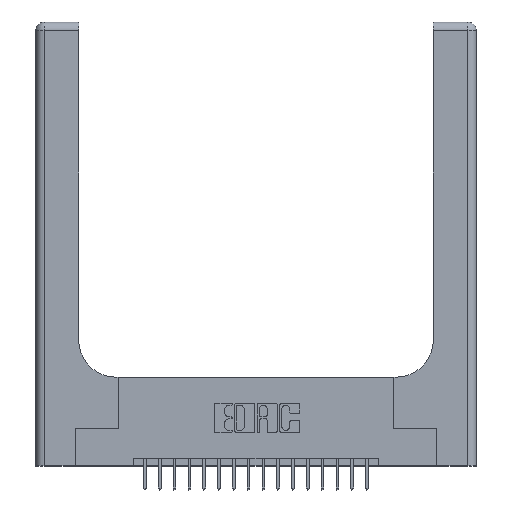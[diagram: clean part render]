
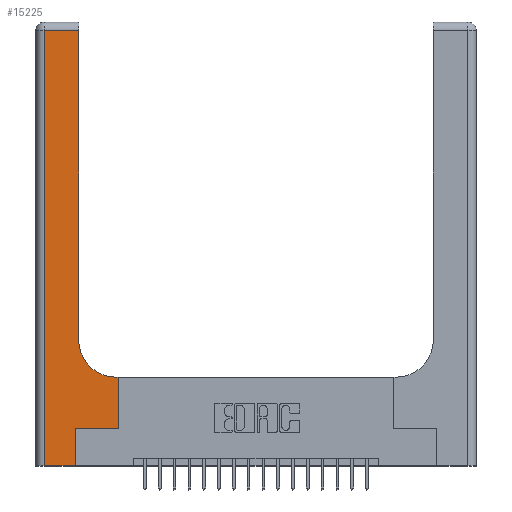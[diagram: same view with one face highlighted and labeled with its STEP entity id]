
A CAD part, top view. The second image highlights one B-rep face of the part: STEP entity #15225.
In plain terms, the highlighted planar face has unit normal (0, 0, 1).
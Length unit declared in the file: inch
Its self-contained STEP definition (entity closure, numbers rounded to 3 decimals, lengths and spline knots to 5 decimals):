
#48 = LINE ( 'NONE', #157, #8401 ) ;
#157 = CARTESIAN_POINT ( 'NONE',  ( 0.06, 3., 0.37 ) ) ;
#583 = CARTESIAN_POINT ( 'NONE',  ( 0.5415, 0.85, 0.37 ) ) ;
#613 = VERTEX_POINT ( 'NONE', #3987 ) ;
#1286 = LINE ( 'NONE', #4008, #18329 ) ;
#1529 = DIRECTION ( 'NONE',  ( 0., 1., 0. ) ) ;
#1548 = CARTESIAN_POINT ( 'NONE',  ( 0.5585, 0.25, 0.37 ) ) ;
#1689 = EDGE_CURVE ( 'NONE', #8178, #613, #48, .T. ) ;
#1707 = AXIS2_PLACEMENT_3D ( 'NONE', #583, #12225, #2245 ) ;
#1746 = CARTESIAN_POINT ( 'NONE',  ( 0., 0., 0.37 ) ) ;
#1817 = DIRECTION ( 'NONE',  ( 0., -1., 0. ) ) ;
#2245 = DIRECTION ( 'NONE',  ( 1., 0., 0. ) ) ;
#2800 = LINE ( 'NONE', #5337, #7235 ) ;
#2855 = EDGE_CURVE ( 'NONE', #16870, #15335, #6807, .T. ) ;
#3178 = CARTESIAN_POINT ( 'NONE',  ( 0.269, 0., 0.37 ) ) ;
#3323 = VECTOR ( 'NONE', #11579, 39.37008 ) ;
#3483 = DIRECTION ( 'NONE',  ( 1., 0., 0. ) ) ;
#3987 = CARTESIAN_POINT ( 'NONE',  ( 0.06, 0., 0.37 ) ) ;
#4008 = CARTESIAN_POINT ( 'NONE',  ( 0.269, 0.25, 0.37 ) ) ;
#4037 = CARTESIAN_POINT ( 'NONE',  ( 0., 3., 0.37 ) ) ;
#4660 = ORIENTED_EDGE ( 'NONE', *, *, #11950, .T. ) ;
#4799 = EDGE_CURVE ( 'NONE', #21310, #8178, #2800, .T. ) ;
#4954 = VERTEX_POINT ( 'NONE', #13936 ) ;
#5124 = ORIENTED_EDGE ( 'NONE', *, *, #17479, .T. ) ;
#5203 = EDGE_CURVE ( 'NONE', #12204, #17050, #15938, .T. ) ;
#5283 = ORIENTED_EDGE ( 'NONE', *, *, #5203, .T. ) ;
#5337 = CARTESIAN_POINT ( 'NONE',  ( 0., 2.94, 0.37 ) ) ;
#5670 = DIRECTION ( 'NONE',  ( 1., 0., 0. ) ) ;
#5701 = PLANE ( 'NONE',  #16734 ) ;
#5713 = CARTESIAN_POINT ( 'NONE',  ( 0.5585, 0.25, 0.37 ) ) ;
#6283 = VECTOR ( 'NONE', #11266, 39.37008 ) ;
#6622 = CARTESIAN_POINT ( 'NONE',  ( 0.2915, 2.94, 0.37 ) ) ;
#6807 = LINE ( 'NONE', #20992, #6283 ) ;
#7235 = VECTOR ( 'NONE', #18490, 39.37008 ) ;
#7390 = DIRECTION ( 'NONE',  ( 0., 0., -1. ) ) ;
#7600 = ORIENTED_EDGE ( 'NONE', *, *, #18216, .T. ) ;
#8178 = VERTEX_POINT ( 'NONE', #20982 ) ;
#8401 = VECTOR ( 'NONE', #1817, 39.37008 ) ;
#8454 = FACE_OUTER_BOUND ( 'NONE', #10889, .T. ) ;
#8678 = VERTEX_POINT ( 'NONE', #5713 ) ;
#9016 = VECTOR ( 'NONE', #14799, 39.37008 ) ;
#9819 = ORIENTED_EDGE ( 'NONE', *, *, #4799, .T. ) ;
#10201 = CARTESIAN_POINT ( 'NONE',  ( 0.5415, 0.6, 0.37 ) ) ;
#10423 = VECTOR ( 'NONE', #1529, 39.37008 ) ;
#10822 = VECTOR ( 'NONE', #3483, 39.37008 ) ;
#10889 = EDGE_LOOP ( 'NONE', ( #5124, #9819, #11384, #4660, #15457, #7600, #12024, #5283, #13872 ) ) ;
#11266 = DIRECTION ( 'NONE',  ( 0., 1., 0. ) ) ;
#11384 = ORIENTED_EDGE ( 'NONE', *, *, #1689, .T. ) ;
#11513 = CARTESIAN_POINT ( 'NONE',  ( 0.2915, 3., 0.37 ) ) ;
#11579 = DIRECTION ( 'NONE',  ( -1., 0., 0. ) ) ;
#11859 = EDGE_CURVE ( 'NONE', #8678, #12204, #21021, .T. ) ;
#11950 = EDGE_CURVE ( 'NONE', #613, #16870, #19522, .T. ) ;
#12024 = ORIENTED_EDGE ( 'NONE', *, *, #11859, .T. ) ;
#12204 = VERTEX_POINT ( 'NONE', #20376 ) ;
#12225 = DIRECTION ( 'NONE',  ( 0., 0., -1. ) ) ;
#12425 = CIRCLE ( 'NONE', #1707, 0.25 ) ;
#12588 = CARTESIAN_POINT ( 'NONE',  ( 0.269, 0.25, 0.37 ) ) ;
#13872 = ORIENTED_EDGE ( 'NONE', *, *, #19265, .T. ) ;
#13936 = CARTESIAN_POINT ( 'NONE',  ( 0.2915, 0.85, 0.37 ) ) ;
#14282 = LINE ( 'NONE', #11513, #10423 ) ;
#14799 = DIRECTION ( 'NONE',  ( 0., 1., 0. ) ) ;
#15225 = ADVANCED_FACE ( 'NONE', ( #8454 ), #5701, .F. ) ;
#15335 = VERTEX_POINT ( 'NONE', #12588 ) ;
#15457 = ORIENTED_EDGE ( 'NONE', *, *, #2855, .T. ) ;
#15938 = LINE ( 'NONE', #21295, #3323 ) ;
#16734 = AXIS2_PLACEMENT_3D ( 'NONE', #4037, #7390, #18847 ) ;
#16870 = VERTEX_POINT ( 'NONE', #3178 ) ;
#17050 = VERTEX_POINT ( 'NONE', #10201 ) ;
#17479 = EDGE_CURVE ( 'NONE', #4954, #21310, #14282, .T. ) ;
#18216 = EDGE_CURVE ( 'NONE', #15335, #8678, #1286, .T. ) ;
#18329 = VECTOR ( 'NONE', #5670, 39.37008 ) ;
#18490 = DIRECTION ( 'NONE',  ( -1., 0., 0. ) ) ;
#18847 = DIRECTION ( 'NONE',  ( -1., 0., 0. ) ) ;
#19265 = EDGE_CURVE ( 'NONE', #17050, #4954, #12425, .T. ) ;
#19522 = LINE ( 'NONE', #1746, #10822 ) ;
#20376 = CARTESIAN_POINT ( 'NONE',  ( 0.5585, 0.6, 0.37 ) ) ;
#20982 = CARTESIAN_POINT ( 'NONE',  ( 0.06, 2.94, 0.37 ) ) ;
#20992 = CARTESIAN_POINT ( 'NONE',  ( 0.269, 0., 0.37 ) ) ;
#21021 = LINE ( 'NONE', #1548, #9016 ) ;
#21295 = CARTESIAN_POINT ( 'NONE',  ( 0.2915, 0.6, 0.37 ) ) ;
#21310 = VERTEX_POINT ( 'NONE', #6622 ) ;
